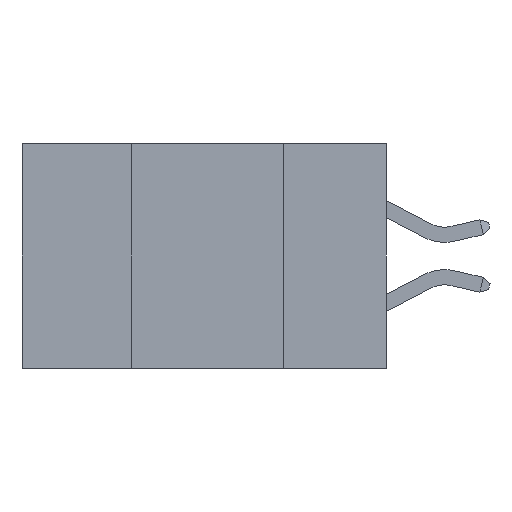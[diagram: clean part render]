
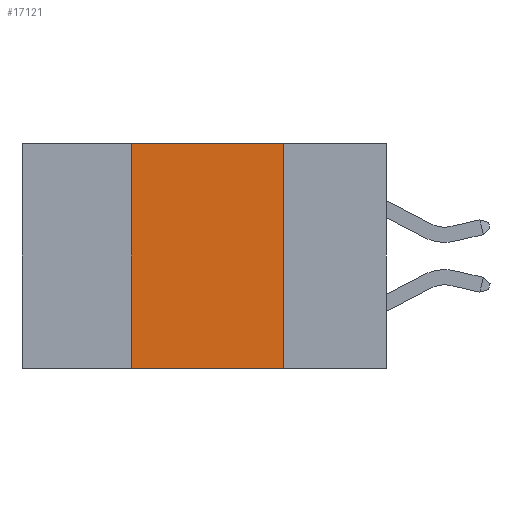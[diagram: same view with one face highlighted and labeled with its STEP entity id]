
A CAD part, left-side view. The second image highlights one B-rep face of the part: STEP entity #17121.
In plain terms, the highlighted planar face has unit normal (-1, 0, 0).
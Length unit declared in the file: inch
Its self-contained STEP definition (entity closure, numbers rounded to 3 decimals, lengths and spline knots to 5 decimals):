
#134 = LINE ( 'NONE', #16794, #3622 ) ;
#158 = CARTESIAN_POINT ( 'NONE',  ( 0., 0.17, -0.37 ) ) ;
#534 = DIRECTION ( 'NONE',  ( 0., -1., 0. ) ) ;
#677 = ORIENTED_EDGE ( 'NONE', *, *, #748, .T. ) ;
#748 = EDGE_CURVE ( 'NONE', #2598, #15578, #12659, .T. ) ;
#1406 = VECTOR ( 'NONE', #10359, 39.37008 ) ;
#2086 = VERTEX_POINT ( 'NONE', #12616 ) ;
#2598 = VERTEX_POINT ( 'NONE', #3830 ) ;
#2809 = DIRECTION ( 'NONE',  ( 0., 0., -1. ) ) ;
#3622 = VECTOR ( 'NONE', #18241, 39.37008 ) ;
#3830 = CARTESIAN_POINT ( 'NONE',  ( 0., 0.42, -0.37 ) ) ;
#4689 = EDGE_CURVE ( 'NONE', #2598, #2086, #134, .T. ) ;
#5384 = CARTESIAN_POINT ( 'NONE',  ( 0., 0.17, 0. ) ) ;
#8170 = ORIENTED_EDGE ( 'NONE', *, *, #15399, .F. ) ;
#8350 = VECTOR ( 'NONE', #534, 39.37008 ) ;
#8595 = EDGE_CURVE ( 'NONE', #2086, #17648, #13051, .T. ) ;
#8629 = CARTESIAN_POINT ( 'NONE',  ( 0., 0.6, 0. ) ) ;
#8891 = CARTESIAN_POINT ( 'NONE',  ( 0., 0.6, 0. ) ) ;
#10359 = DIRECTION ( 'NONE',  ( 0., -1., 0. ) ) ;
#11560 = DIRECTION ( 'NONE',  ( 1., 0., 0. ) ) ;
#11719 = VECTOR ( 'NONE', #11875, 39.37008 ) ;
#11875 = DIRECTION ( 'NONE',  ( 0., 0., -1. ) ) ;
#12101 = FACE_OUTER_BOUND ( 'NONE', #18340, .T. ) ;
#12616 = CARTESIAN_POINT ( 'NONE',  ( 0., 0.42, 0. ) ) ;
#12659 = LINE ( 'NONE', #17965, #8350 ) ;
#12940 = PLANE ( 'NONE',  #14113 ) ;
#13051 = LINE ( 'NONE', #8891, #1406 ) ;
#13091 = LINE ( 'NONE', #158, #11719 ) ;
#13143 = ORIENTED_EDGE ( 'NONE', *, *, #8595, .F. ) ;
#14113 = AXIS2_PLACEMENT_3D ( 'NONE', #8629, #11560, #2809 ) ;
#15172 = ORIENTED_EDGE ( 'NONE', *, *, #4689, .F. ) ;
#15399 = EDGE_CURVE ( 'NONE', #17648, #15578, #13091, .T. ) ;
#15578 = VERTEX_POINT ( 'NONE', #17976 ) ;
#16794 = CARTESIAN_POINT ( 'NONE',  ( 0., 0.42, -0.37 ) ) ;
#17121 = ADVANCED_FACE ( 'NONE', ( #12101 ), #12940, .F. ) ;
#17648 = VERTEX_POINT ( 'NONE', #5384 ) ;
#17965 = CARTESIAN_POINT ( 'NONE',  ( 0., 0.6, -0.37 ) ) ;
#17976 = CARTESIAN_POINT ( 'NONE',  ( 0., 0.17, -0.37 ) ) ;
#18241 = DIRECTION ( 'NONE',  ( 0., 0., 1. ) ) ;
#18340 = EDGE_LOOP ( 'NONE', ( #8170, #13143, #15172, #677 ) ) ;
